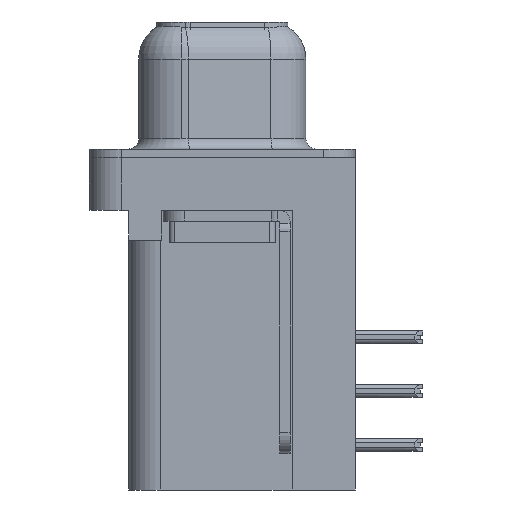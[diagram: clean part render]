
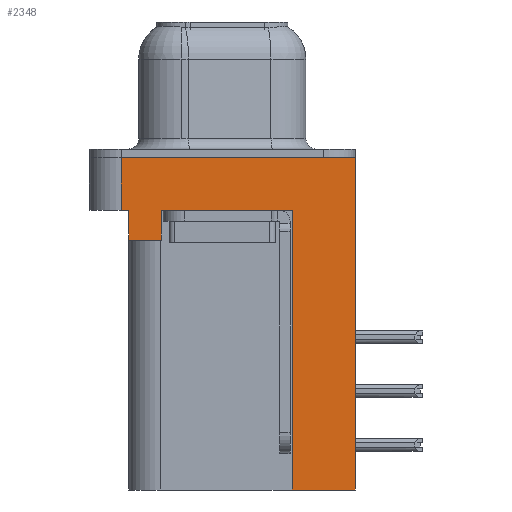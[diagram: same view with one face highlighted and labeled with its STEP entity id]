
A CAD part, left-side view. The second image highlights one B-rep face of the part: STEP entity #2348.
In plain terms, the highlighted planar face has unit normal (-1, 0, 0).
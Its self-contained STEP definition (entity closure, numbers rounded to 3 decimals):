
#167 = VECTOR ( 'NONE', #32067, 1000. ) ;
#685 = VECTOR ( 'NONE', #15896, 1000. ) ;
#726 = CARTESIAN_POINT ( 'NONE',  ( -2.935, 2.895, -2.5 ) ) ;
#1280 = CARTESIAN_POINT ( 'NONE',  ( -2.935, -6.275, -2.5 ) ) ;
#1880 = VECTOR ( 'NONE', #32652, 1000. ) ;
#2332 = ORIENTED_EDGE ( 'NONE', *, *, #16826, .T. ) ;
#2348 = ADVANCED_FACE ( 'NONE', ( #25011 ), #22952, .T. ) ;
#2901 = ORIENTED_EDGE ( 'NONE', *, *, #34277, .F. ) ;
#3476 = VECTOR ( 'NONE', #32344, 1000. ) ;
#3868 = DIRECTION ( 'NONE',  ( 0., -1., 0. ) ) ;
#5062 = EDGE_CURVE ( 'NONE', #34768, #14602, #26220, .T. ) ;
#6069 = VERTEX_POINT ( 'NONE', #36569 ) ;
#6482 = CARTESIAN_POINT ( 'NONE',  ( -2.935, -6.275, 0. ) ) ;
#6672 = CARTESIAN_POINT ( 'NONE',  ( -2.935, 4.425, -3.9 ) ) ;
#7763 = LINE ( 'NONE', #35014, #167 ) ;
#9104 = VERTEX_POINT ( 'NONE', #22834 ) ;
#9148 = ORIENTED_EDGE ( 'NONE', *, *, #35095, .F. ) ;
#9427 = CARTESIAN_POINT ( 'NONE',  ( -2.935, -3.295, -15.7 ) ) ;
#9459 = LINE ( 'NONE', #1280, #1880 ) ;
#9908 = CARTESIAN_POINT ( 'NONE',  ( -2.935, -6.275, -2.5 ) ) ;
#11271 = ORIENTED_EDGE ( 'NONE', *, *, #36093, .F. ) ;
#11551 = CARTESIAN_POINT ( 'NONE',  ( -2.935, 4.425, -3.9 ) ) ;
#11905 = CARTESIAN_POINT ( 'NONE',  ( -2.935, -6.275, -15.7 ) ) ;
#12393 = DIRECTION ( 'NONE',  ( 0., 0., 1. ) ) ;
#13018 = CARTESIAN_POINT ( 'NONE',  ( -2.935, -6.275, -2.5 ) ) ;
#13214 = VECTOR ( 'NONE', #17313, 1000. ) ;
#13343 = LINE ( 'NONE', #21779, #34121 ) ;
#13476 = ORIENTED_EDGE ( 'NONE', *, *, #28906, .F. ) ;
#13496 = VECTOR ( 'NONE', #21697, 1000. ) ;
#14509 = ORIENTED_EDGE ( 'NONE', *, *, #5062, .F. ) ;
#14518 = LINE ( 'NONE', #35973, #15417 ) ;
#14602 = VERTEX_POINT ( 'NONE', #33837 ) ;
#15417 = VECTOR ( 'NONE', #24829, 1000. ) ;
#15896 = DIRECTION ( 'NONE',  ( 0., -1., 0. ) ) ;
#16826 = EDGE_CURVE ( 'NONE', #22831, #23885, #16890, .T. ) ;
#16890 = LINE ( 'NONE', #13018, #685 ) ;
#17313 = DIRECTION ( 'NONE',  ( 0., 0., 1. ) ) ;
#18681 = CARTESIAN_POINT ( 'NONE',  ( -2.935, 4.425, -2.5 ) ) ;
#18871 = DIRECTION ( 'NONE',  ( 0., -1., 0. ) ) ;
#18966 = VECTOR ( 'NONE', #12393, 1000. ) ;
#19475 = ORIENTED_EDGE ( 'NONE', *, *, #35890, .F. ) ;
#20125 = VERTEX_POINT ( 'NONE', #11905 ) ;
#20589 = CARTESIAN_POINT ( 'NONE',  ( -2.935, 4.425, -3.9 ) ) ;
#21595 = VERTEX_POINT ( 'NONE', #20589 ) ;
#21697 = DIRECTION ( 'NONE',  ( 0., 0., 1. ) ) ;
#21725 = ORIENTED_EDGE ( 'NONE', *, *, #30395, .T. ) ;
#21779 = CARTESIAN_POINT ( 'NONE',  ( -2.935, -6.275, -2.5 ) ) ;
#21896 = ORIENTED_EDGE ( 'NONE', *, *, #22258, .T. ) ;
#22258 = EDGE_CURVE ( 'NONE', #28775, #22831, #36025, .T. ) ;
#22721 = ORIENTED_EDGE ( 'NONE', *, *, #36550, .T. ) ;
#22831 = VERTEX_POINT ( 'NONE', #726 ) ;
#22834 = CARTESIAN_POINT ( 'NONE',  ( -2.935, 4.775, -2.5 ) ) ;
#22952 = PLANE ( 'NONE',  #25280 ) ;
#23438 = CARTESIAN_POINT ( 'NONE',  ( -2.935, 4.775, 0. ) ) ;
#23885 = VERTEX_POINT ( 'NONE', #32414 ) ;
#24522 = CARTESIAN_POINT ( 'NONE',  ( -2.935, 2.895, -3.9 ) ) ;
#24829 = DIRECTION ( 'NONE',  ( 0., 1., 0. ) ) ;
#25011 = FACE_OUTER_BOUND ( 'NONE', #27161, .T. ) ;
#25280 = AXIS2_PLACEMENT_3D ( 'NONE', #9908, #35858, #35772 ) ;
#25342 = VECTOR ( 'NONE', #3868, 1000. ) ;
#25421 = LINE ( 'NONE', #6672, #3476 ) ;
#26206 = CARTESIAN_POINT ( 'NONE',  ( -2.935, 2.895, -3.9 ) ) ;
#26220 = LINE ( 'NONE', #6482, #25342 ) ;
#27161 = EDGE_LOOP ( 'NONE', ( #14509, #2901, #21725, #9148, #13476, #21896, #2332, #19475, #11271, #22721 ) ) ;
#28286 = LINE ( 'NONE', #11551, #13214 ) ;
#28775 = VERTEX_POINT ( 'NONE', #26206 ) ;
#28906 = EDGE_CURVE ( 'NONE', #28775, #21595, #25421, .T. ) ;
#29872 = VERTEX_POINT ( 'NONE', #18681 ) ;
#30395 = EDGE_CURVE ( 'NONE', #9104, #29872, #13343, .T. ) ;
#32067 = DIRECTION ( 'NONE',  ( 0., 0., 1. ) ) ;
#32344 = DIRECTION ( 'NONE',  ( 0., 1., 0. ) ) ;
#32414 = CARTESIAN_POINT ( 'NONE',  ( -2.935, -3.295, -2.5 ) ) ;
#32652 = DIRECTION ( 'NONE',  ( 0., 0., 1. ) ) ;
#33837 = CARTESIAN_POINT ( 'NONE',  ( -2.935, -6.275, 0. ) ) ;
#34121 = VECTOR ( 'NONE', #18871, 1000. ) ;
#34277 = EDGE_CURVE ( 'NONE', #9104, #34768, #7763, .T. ) ;
#34768 = VERTEX_POINT ( 'NONE', #23438 ) ;
#34851 = LINE ( 'NONE', #9427, #18966 ) ;
#35014 = CARTESIAN_POINT ( 'NONE',  ( -2.935, 4.775, -2.5 ) ) ;
#35095 = EDGE_CURVE ( 'NONE', #21595, #29872, #28286, .T. ) ;
#35772 = DIRECTION ( 'NONE',  ( 0., 0., 1. ) ) ;
#35858 = DIRECTION ( 'NONE',  ( -1., 0., 0. ) ) ;
#35890 = EDGE_CURVE ( 'NONE', #6069, #23885, #34851, .T. ) ;
#35973 = CARTESIAN_POINT ( 'NONE',  ( -2.935, -3.295, -15.7 ) ) ;
#36025 = LINE ( 'NONE', #24522, #13496 ) ;
#36093 = EDGE_CURVE ( 'NONE', #20125, #6069, #14518, .T. ) ;
#36550 = EDGE_CURVE ( 'NONE', #20125, #14602, #9459, .T. ) ;
#36569 = CARTESIAN_POINT ( 'NONE',  ( -2.935, -3.295, -15.7 ) ) ;
